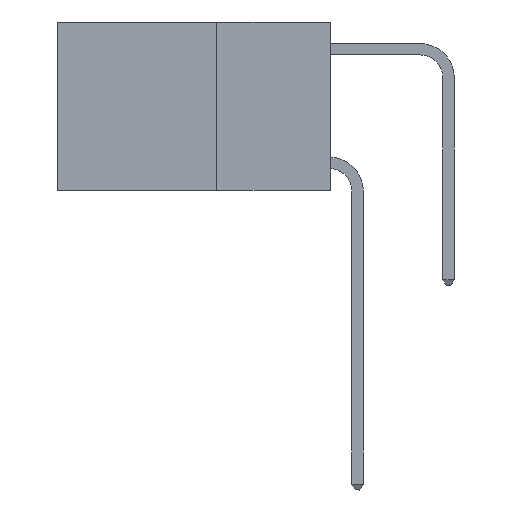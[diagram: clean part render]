
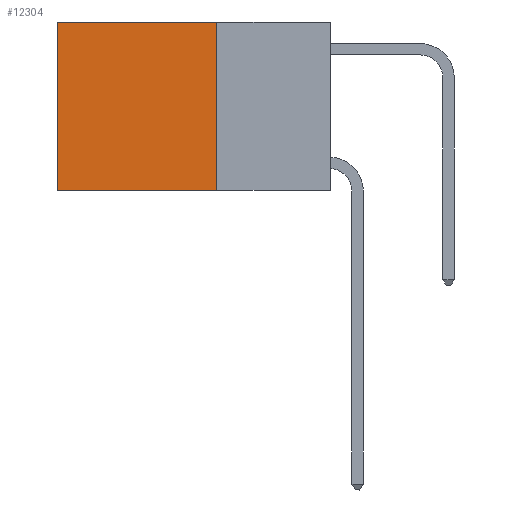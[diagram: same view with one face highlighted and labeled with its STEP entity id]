
A CAD part, left-side view. The second image highlights one B-rep face of the part: STEP entity #12304.
In plain terms, the highlighted planar face has unit normal (-1, 0, 0).
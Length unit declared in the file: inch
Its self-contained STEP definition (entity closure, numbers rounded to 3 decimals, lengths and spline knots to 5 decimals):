
#74 = EDGE_LOOP ( 'NONE', ( #10939, #3477, #816, #4770 ) ) ;
#613 = LINE ( 'NONE', #5646, #12616 ) ;
#746 = VERTEX_POINT ( 'NONE', #10636 ) ;
#816 = ORIENTED_EDGE ( 'NONE', *, *, #3587, .F. ) ;
#1504 = EDGE_CURVE ( 'NONE', #5929, #5149, #3708, .T. ) ;
#3060 = AXIS2_PLACEMENT_3D ( 'NONE', #3290, #4516, #12802 ) ;
#3177 = VERTEX_POINT ( 'NONE', #9704 ) ;
#3290 = CARTESIAN_POINT ( 'NONE',  ( 0.2625, 0.25, 0. ) ) ;
#3477 = ORIENTED_EDGE ( 'NONE', *, *, #1504, .F. ) ;
#3587 = EDGE_CURVE ( 'NONE', #3177, #5929, #6777, .T. ) ;
#3708 = LINE ( 'NONE', #10718, #9726 ) ;
#3974 = DIRECTION ( 'NONE',  ( 0., 1., 0. ) ) ;
#4516 = DIRECTION ( 'NONE',  ( 1., 0., 0. ) ) ;
#4770 = ORIENTED_EDGE ( 'NONE', *, *, #11004, .T. ) ;
#4998 = CARTESIAN_POINT ( 'NONE',  ( 0.2625, 0.6, -0.37 ) ) ;
#5149 = VERTEX_POINT ( 'NONE', #4998 ) ;
#5646 = CARTESIAN_POINT ( 'NONE',  ( 0.2625, 0.6, 0. ) ) ;
#5725 = LINE ( 'NONE', #9953, #11715 ) ;
#5929 = VERTEX_POINT ( 'NONE', #11199 ) ;
#6777 = LINE ( 'NONE', #10430, #9607 ) ;
#9224 = DIRECTION ( 'NONE',  ( 0., 0., -1. ) ) ;
#9607 = VECTOR ( 'NONE', #9224, 39.37008 ) ;
#9704 = CARTESIAN_POINT ( 'NONE',  ( 0.2625, 0.25, 0. ) ) ;
#9726 = VECTOR ( 'NONE', #13075, 39.37008 ) ;
#9953 = CARTESIAN_POINT ( 'NONE',  ( 0.2625, 0.25, 0. ) ) ;
#10430 = CARTESIAN_POINT ( 'NONE',  ( 0.2625, 0.25, 0. ) ) ;
#10478 = PLANE ( 'NONE',  #3060 ) ;
#10636 = CARTESIAN_POINT ( 'NONE',  ( 0.2625, 0.6, 0. ) ) ;
#10709 = EDGE_CURVE ( 'NONE', #746, #5149, #613, .T. ) ;
#10718 = CARTESIAN_POINT ( 'NONE',  ( 0.2625, 0.25, -0.37 ) ) ;
#10939 = ORIENTED_EDGE ( 'NONE', *, *, #10709, .T. ) ;
#11004 = EDGE_CURVE ( 'NONE', #3177, #746, #5725, .T. ) ;
#11199 = CARTESIAN_POINT ( 'NONE',  ( 0.2625, 0.25, -0.37 ) ) ;
#11715 = VECTOR ( 'NONE', #3974, 39.37008 ) ;
#11871 = FACE_OUTER_BOUND ( 'NONE', #74, .T. ) ;
#12304 = ADVANCED_FACE ( 'NONE', ( #11871 ), #10478, .F. ) ;
#12616 = VECTOR ( 'NONE', #12754, 39.37008 ) ;
#12754 = DIRECTION ( 'NONE',  ( 0., 0., -1. ) ) ;
#12802 = DIRECTION ( 'NONE',  ( 0., 0., -1. ) ) ;
#13075 = DIRECTION ( 'NONE',  ( 0., 1., 0. ) ) ;
